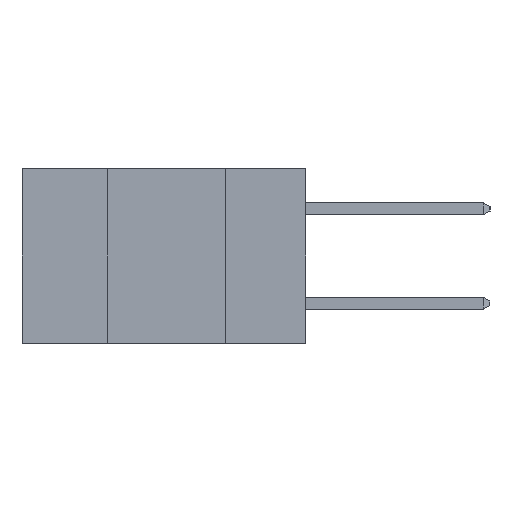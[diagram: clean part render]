
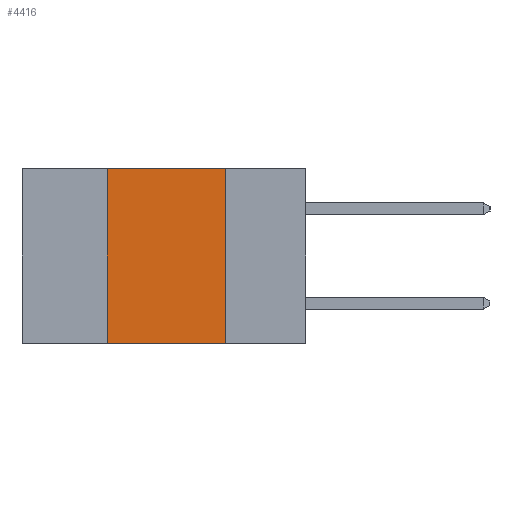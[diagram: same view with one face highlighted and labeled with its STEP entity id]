
A CAD part, left-side view. The second image highlights one B-rep face of the part: STEP entity #4416.
In plain terms, the highlighted planar face has unit normal (-1, 0, 0).
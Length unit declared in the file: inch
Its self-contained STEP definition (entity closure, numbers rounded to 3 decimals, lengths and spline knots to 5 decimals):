
#614 = VERTEX_POINT ( 'NONE', #11442 ) ;
#987 = VERTEX_POINT ( 'NONE', #6965 ) ;
#993 = EDGE_CURVE ( 'NONE', #614, #3831, #1503, .T. ) ;
#1099 = ORIENTED_EDGE ( 'NONE', *, *, #13237, .T. ) ;
#1503 = LINE ( 'NONE', #5728, #8538 ) ;
#1642 = DIRECTION ( 'NONE',  ( 0., 0., -1. ) ) ;
#1911 = CARTESIAN_POINT ( 'NONE',  ( 0., 0.6, 0. ) ) ;
#1930 = ORIENTED_EDGE ( 'NONE', *, *, #993, .F. ) ;
#2058 = CARTESIAN_POINT ( 'NONE',  ( 0., 0.17, -0.37 ) ) ;
#2507 = LINE ( 'NONE', #12041, #6809 ) ;
#2678 = DIRECTION ( 'NONE',  ( 0., 0., 1. ) ) ;
#2967 = FACE_OUTER_BOUND ( 'NONE', #3418, .T. ) ;
#3418 = EDGE_LOOP ( 'NONE', ( #3906, #9408, #1930, #1099 ) ) ;
#3655 = VECTOR ( 'NONE', #10540, 39.37008 ) ;
#3831 = VERTEX_POINT ( 'NONE', #7901 ) ;
#3906 = ORIENTED_EDGE ( 'NONE', *, *, #12704, .F. ) ;
#4416 = ADVANCED_FACE ( 'NONE', ( #2967 ), #13613, .F. ) ;
#4971 = VERTEX_POINT ( 'NONE', #13230 ) ;
#5728 = CARTESIAN_POINT ( 'NONE',  ( 0., 0.42, -0.37 ) ) ;
#5927 = LINE ( 'NONE', #8291, #10006 ) ;
#6121 = EDGE_CURVE ( 'NONE', #3831, #4971, #5927, .T. ) ;
#6219 = DIRECTION ( 'NONE',  ( 1., 0., 0. ) ) ;
#6295 = LINE ( 'NONE', #2058, #3655 ) ;
#6809 = VECTOR ( 'NONE', #13369, 39.37008 ) ;
#6965 = CARTESIAN_POINT ( 'NONE',  ( 0., 0.17, -0.37 ) ) ;
#7901 = CARTESIAN_POINT ( 'NONE',  ( 0., 0.42, 0. ) ) ;
#8291 = CARTESIAN_POINT ( 'NONE',  ( 0., 0.6, 0. ) ) ;
#8538 = VECTOR ( 'NONE', #2678, 39.37008 ) ;
#9408 = ORIENTED_EDGE ( 'NONE', *, *, #6121, .F. ) ;
#10006 = VECTOR ( 'NONE', #12542, 39.37008 ) ;
#10540 = DIRECTION ( 'NONE',  ( 0., 0., -1. ) ) ;
#11442 = CARTESIAN_POINT ( 'NONE',  ( 0., 0.42, -0.37 ) ) ;
#11505 = AXIS2_PLACEMENT_3D ( 'NONE', #1911, #6219, #1642 ) ;
#12041 = CARTESIAN_POINT ( 'NONE',  ( 0., 0.6, -0.37 ) ) ;
#12542 = DIRECTION ( 'NONE',  ( 0., -1., 0. ) ) ;
#12704 = EDGE_CURVE ( 'NONE', #4971, #987, #6295, .T. ) ;
#13230 = CARTESIAN_POINT ( 'NONE',  ( 0., 0.17, 0. ) ) ;
#13237 = EDGE_CURVE ( 'NONE', #614, #987, #2507, .T. ) ;
#13369 = DIRECTION ( 'NONE',  ( 0., -1., 0. ) ) ;
#13613 = PLANE ( 'NONE',  #11505 ) ;
